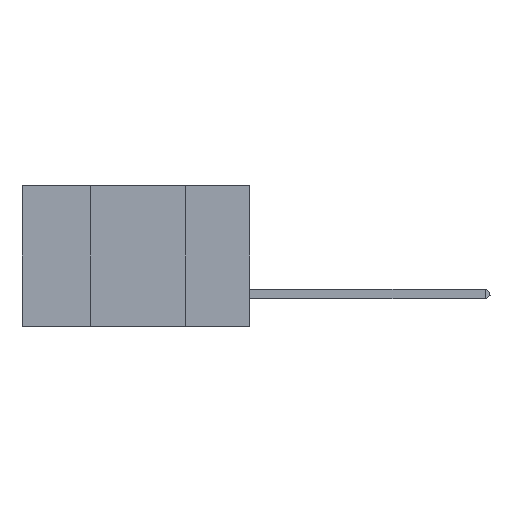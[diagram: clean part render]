
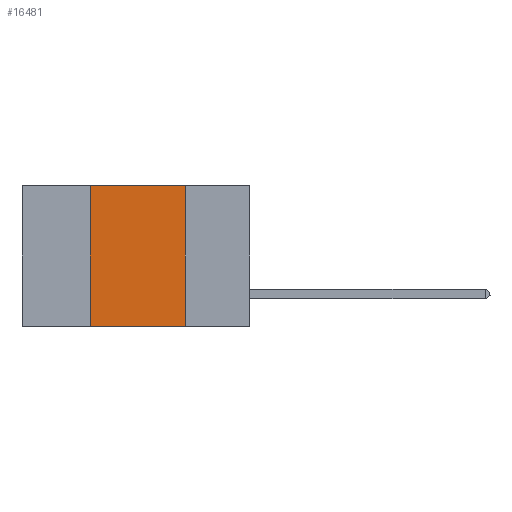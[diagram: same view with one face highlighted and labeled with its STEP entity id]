
A CAD part, left-side view. The second image highlights one B-rep face of the part: STEP entity #16481.
In plain terms, the highlighted planar face has unit normal (-1, 0, 0).
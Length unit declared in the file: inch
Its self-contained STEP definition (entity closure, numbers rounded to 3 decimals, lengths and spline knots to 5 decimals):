
#175 = CARTESIAN_POINT ( 'NONE',  ( 0., 0.42, -0.37 ) ) ;
#1965 = CARTESIAN_POINT ( 'NONE',  ( 0., 0.17, -0.37 ) ) ;
#3335 = EDGE_LOOP ( 'NONE', ( #29899, #15249, #37979, #17290 ) ) ;
#4002 = DIRECTION ( 'NONE',  ( 1., 0., 0. ) ) ;
#9730 = CARTESIAN_POINT ( 'NONE',  ( 0., 0.42, 0. ) ) ;
#13894 = CARTESIAN_POINT ( 'NONE',  ( 0., 0.17, 0. ) ) ;
#13918 = VERTEX_POINT ( 'NONE', #1965 ) ;
#15249 = ORIENTED_EDGE ( 'NONE', *, *, #45393, .F. ) ;
#15392 = VECTOR ( 'NONE', #40731, 39.37008 ) ;
#15552 = LINE ( 'NONE', #27460, #26348 ) ;
#16481 = ADVANCED_FACE ( 'NONE', ( #47303 ), #42070, .F. ) ;
#16763 = VERTEX_POINT ( 'NONE', #39532 ) ;
#17290 = ORIENTED_EDGE ( 'NONE', *, *, #37539, .T. ) ;
#19086 = AXIS2_PLACEMENT_3D ( 'NONE', #34787, #4002, #45763 ) ;
#19182 = EDGE_CURVE ( 'NONE', #43580, #16763, #45545, .T. ) ;
#20977 = VECTOR ( 'NONE', #40346, 39.37008 ) ;
#26348 = VECTOR ( 'NONE', #46490, 39.37008 ) ;
#27460 = CARTESIAN_POINT ( 'NONE',  ( 0., 0.6, 0. ) ) ;
#29899 = ORIENTED_EDGE ( 'NONE', *, *, #33175, .F. ) ;
#32504 = CARTESIAN_POINT ( 'NONE',  ( 0., 0.6, -0.37 ) ) ;
#33175 = EDGE_CURVE ( 'NONE', #49162, #13918, #38383, .T. ) ;
#34787 = CARTESIAN_POINT ( 'NONE',  ( 0., 0.6, 0. ) ) ;
#36011 = DIRECTION ( 'NONE',  ( 0., -1., 0. ) ) ;
#36268 = CARTESIAN_POINT ( 'NONE',  ( 0., 0.17, 0. ) ) ;
#37539 = EDGE_CURVE ( 'NONE', #43580, #13918, #44719, .T. ) ;
#37979 = ORIENTED_EDGE ( 'NONE', *, *, #19182, .F. ) ;
#38383 = LINE ( 'NONE', #13894, #20977 ) ;
#39532 = CARTESIAN_POINT ( 'NONE',  ( 0., 0.42, 0. ) ) ;
#40346 = DIRECTION ( 'NONE',  ( 0., 0., -1. ) ) ;
#40731 = DIRECTION ( 'NONE',  ( 0., 0., 1. ) ) ;
#41708 = VECTOR ( 'NONE', #36011, 39.37008 ) ;
#42070 = PLANE ( 'NONE',  #19086 ) ;
#43580 = VERTEX_POINT ( 'NONE', #175 ) ;
#44719 = LINE ( 'NONE', #32504, #41708 ) ;
#45393 = EDGE_CURVE ( 'NONE', #16763, #49162, #15552, .T. ) ;
#45545 = LINE ( 'NONE', #9730, #15392 ) ;
#45763 = DIRECTION ( 'NONE',  ( 0., 0., -1. ) ) ;
#46490 = DIRECTION ( 'NONE',  ( 0., -1., 0. ) ) ;
#47303 = FACE_OUTER_BOUND ( 'NONE', #3335, .T. ) ;
#49162 = VERTEX_POINT ( 'NONE', #36268 ) ;
